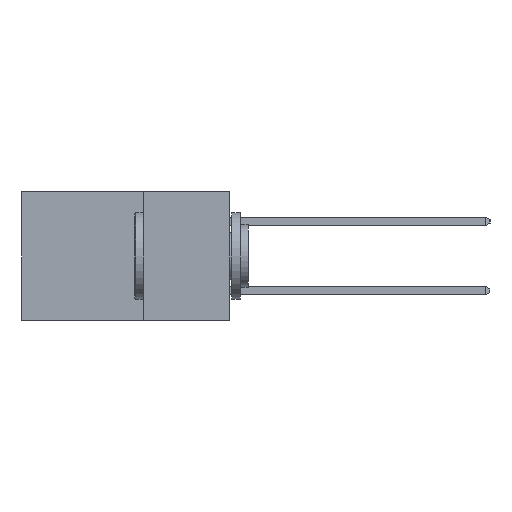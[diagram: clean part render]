
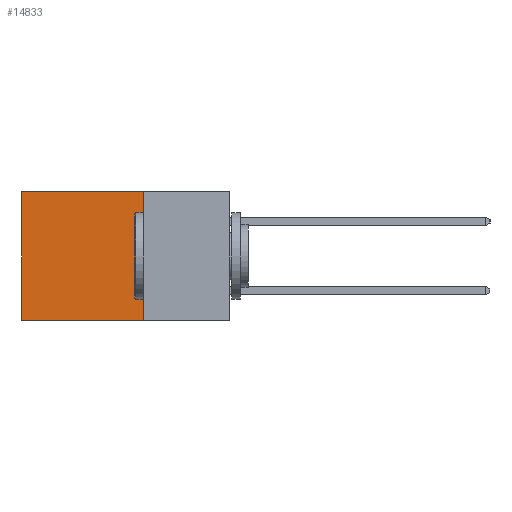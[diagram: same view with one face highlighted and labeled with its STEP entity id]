
A CAD part, left-side view. The second image highlights one B-rep face of the part: STEP entity #14833.
In plain terms, the highlighted planar face has unit normal (-1, 0, 0).
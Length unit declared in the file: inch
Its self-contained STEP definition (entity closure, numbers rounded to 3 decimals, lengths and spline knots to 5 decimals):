
#1081 = VERTEX_POINT ( 'NONE', #10844 ) ;
#1601 = PLANE ( 'NONE',  #3647 ) ;
#1920 = VECTOR ( 'NONE', #22695, 39.37008 ) ;
#2769 = CARTESIAN_POINT ( 'NONE',  ( 0.2615, 0.25, 0. ) ) ;
#3430 = DIRECTION ( 'NONE',  ( 0., 0., -1. ) ) ;
#3647 = AXIS2_PLACEMENT_3D ( 'NONE', #19808, #14381, #3430 ) ;
#3960 = CARTESIAN_POINT ( 'NONE',  ( 0.2615, 0.25, -0.37 ) ) ;
#4325 = EDGE_LOOP ( 'NONE', ( #5677, #23139, #8695, #18961 ) ) ;
#4444 = CARTESIAN_POINT ( 'NONE',  ( 0.2615, 0.25, -0.37 ) ) ;
#4774 = LINE ( 'NONE', #6135, #23580 ) ;
#5270 = CARTESIAN_POINT ( 'NONE',  ( 0.2615, 0.6, 0. ) ) ;
#5401 = VERTEX_POINT ( 'NONE', #5270 ) ;
#5677 = ORIENTED_EDGE ( 'NONE', *, *, #20663, .T. ) ;
#5826 = EDGE_CURVE ( 'NONE', #17078, #1081, #15944, .T. ) ;
#6135 = CARTESIAN_POINT ( 'NONE',  ( 0.2615, 0.6, -0.37 ) ) ;
#7036 = DIRECTION ( 'NONE',  ( 0., 0., -1. ) ) ;
#8106 = EDGE_CURVE ( 'NONE', #21444, #5401, #11825, .T. ) ;
#8695 = ORIENTED_EDGE ( 'NONE', *, *, #22371, .F. ) ;
#8873 = CARTESIAN_POINT ( 'NONE',  ( 0.2615, 0.25, -0.37 ) ) ;
#9253 = FACE_OUTER_BOUND ( 'NONE', #4325, .T. ) ;
#9806 = DIRECTION ( 'NONE',  ( 0., 0., -1. ) ) ;
#10844 = CARTESIAN_POINT ( 'NONE',  ( 0.2615, 0.6, -0.37 ) ) ;
#10871 = LINE ( 'NONE', #8873, #11453 ) ;
#11453 = VECTOR ( 'NONE', #7036, 39.37008 ) ;
#11825 = LINE ( 'NONE', #23397, #20995 ) ;
#14381 = DIRECTION ( 'NONE',  ( 1., 0., 0. ) ) ;
#14833 = ADVANCED_FACE ( 'NONE', ( #9253 ), #1601, .F. ) ;
#15944 = LINE ( 'NONE', #4444, #1920 ) ;
#17078 = VERTEX_POINT ( 'NONE', #3960 ) ;
#18961 = ORIENTED_EDGE ( 'NONE', *, *, #8106, .T. ) ;
#19808 = CARTESIAN_POINT ( 'NONE',  ( 0.2615, 0.25, -0.37 ) ) ;
#20663 = EDGE_CURVE ( 'NONE', #5401, #1081, #4774, .T. ) ;
#20995 = VECTOR ( 'NONE', #23469, 39.37008 ) ;
#21444 = VERTEX_POINT ( 'NONE', #2769 ) ;
#22371 = EDGE_CURVE ( 'NONE', #21444, #17078, #10871, .T. ) ;
#22695 = DIRECTION ( 'NONE',  ( 0., 1., 0. ) ) ;
#23139 = ORIENTED_EDGE ( 'NONE', *, *, #5826, .F. ) ;
#23397 = CARTESIAN_POINT ( 'NONE',  ( 0.2615, 0.25, 0. ) ) ;
#23469 = DIRECTION ( 'NONE',  ( 0., 1., 0. ) ) ;
#23580 = VECTOR ( 'NONE', #9806, 39.37008 ) ;
